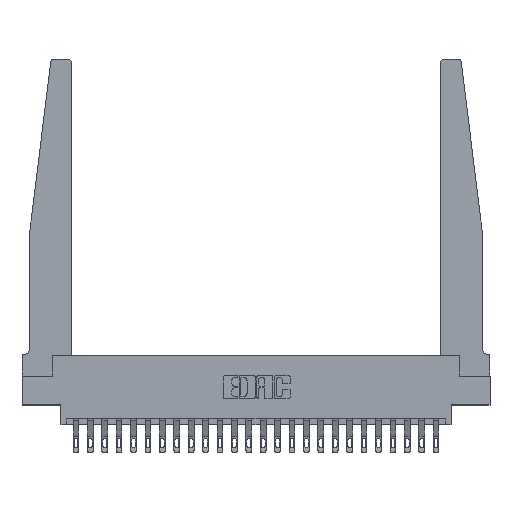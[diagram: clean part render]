
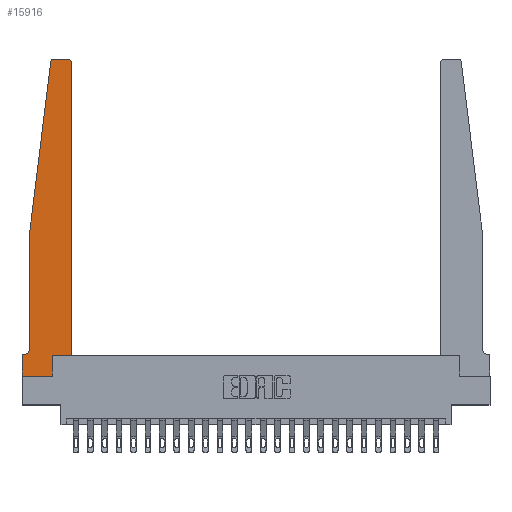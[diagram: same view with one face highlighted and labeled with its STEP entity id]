
A CAD part, top view. The second image highlights one B-rep face of the part: STEP entity #15916.
In plain terms, the highlighted planar face has unit normal (0, 0, 1).
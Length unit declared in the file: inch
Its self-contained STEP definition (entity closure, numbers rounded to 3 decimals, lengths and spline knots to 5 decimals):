
#28 = CARTESIAN_POINT ( 'NONE',  ( 0.015, 0.1875, 0.37 ) ) ;
#70 = LINE ( 'NONE', #19010, #5690 ) ;
#194 = DIRECTION ( 'NONE',  ( 0., 1., 0. ) ) ;
#240 = DIRECTION ( 'NONE',  ( 1., 0., 0. ) ) ;
#373 = ORIENTED_EDGE ( 'NONE', *, *, #10259, .T. ) ;
#909 = CIRCLE ( 'NONE', #4108, 0.05 ) ;
#1382 = CARTESIAN_POINT ( 'NONE',  ( 0.015, 0.2375, 0.37 ) ) ;
#1850 = LINE ( 'NONE', #20656, #7805 ) ;
#1872 = AXIS2_PLACEMENT_3D ( 'NONE', #8564, #6312, #14222 ) ;
#1913 = VECTOR ( 'NONE', #11447, 39.37008 ) ;
#2005 = VECTOR ( 'NONE', #15147, 39.37008 ) ;
#2633 = CIRCLE ( 'NONE', #9837, 0.03 ) ;
#2907 = FACE_OUTER_BOUND ( 'NONE', #6926, .T. ) ;
#2997 = CARTESIAN_POINT ( 'NONE',  ( 0.065, 0.2375, 0.37 ) ) ;
#3524 = CARTESIAN_POINT ( 'NONE',  ( 0., 0.1875, 0.37 ) ) ;
#4108 = AXIS2_PLACEMENT_3D ( 'NONE', #1382, #23730, #6535 ) ;
#4109 = EDGE_CURVE ( 'NONE', #15011, #24772, #13547, .T. ) ;
#5056 = VERTEX_POINT ( 'NONE', #17362 ) ;
#5690 = VECTOR ( 'NONE', #194, 39.37008 ) ;
#5766 = CARTESIAN_POINT ( 'NONE',  ( 0.27653, 2.72, 0.37 ) ) ;
#6125 = CARTESIAN_POINT ( 'NONE',  ( 0.395, 2.75, 0.37 ) ) ;
#6137 = VECTOR ( 'NONE', #12369, 39.37008 ) ;
#6312 = DIRECTION ( 'NONE',  ( 0., 0., 1. ) ) ;
#6467 = LINE ( 'NONE', #10232, #6137 ) ;
#6535 = DIRECTION ( 'NONE',  ( -1., 0., 0. ) ) ;
#6581 = ORIENTED_EDGE ( 'NONE', *, *, #11618, .T. ) ;
#6617 = CARTESIAN_POINT ( 'NONE',  ( 0.27653, 2.75, 0.37 ) ) ;
#6688 = EDGE_CURVE ( 'NONE', #13780, #5056, #14677, .T. ) ;
#6808 = CARTESIAN_POINT ( 'NONE',  ( 0.065, 1.25, 0.37 ) ) ;
#6926 = EDGE_LOOP ( 'NONE', ( #17609, #11077, #15080, #15619, #17497, #6581, #24684, #23770, #11872, #17098, #373, #19827 ) ) ;
#7206 = CARTESIAN_POINT ( 'NONE',  ( 0.425, 0.18, 0.37 ) ) ;
#7258 = EDGE_CURVE ( 'NONE', #12325, #13549, #1850, .T. ) ;
#7486 = CARTESIAN_POINT ( 'NONE',  ( 0.395, 2.72, 0.37 ) ) ;
#7602 = DIRECTION ( 'NONE',  ( -1., 0., 0. ) ) ;
#7733 = CARTESIAN_POINT ( 'NONE',  ( 0., 0., 0.37 ) ) ;
#7805 = VECTOR ( 'NONE', #11148, 39.37008 ) ;
#8400 = VERTEX_POINT ( 'NONE', #12075 ) ;
#8454 = CARTESIAN_POINT ( 'NONE',  ( 0.2605, 0.18, 0.37 ) ) ;
#8564 = CARTESIAN_POINT ( 'NONE',  ( 0., 0.1875, 0.37 ) ) ;
#8836 = VECTOR ( 'NONE', #7602, 39.37008 ) ;
#9041 = AXIS2_PLACEMENT_3D ( 'NONE', #5766, #12849, #10713 ) ;
#9180 = EDGE_CURVE ( 'NONE', #5056, #12325, #16848, .T. ) ;
#9837 = AXIS2_PLACEMENT_3D ( 'NONE', #7486, #13258, #19990 ) ;
#10232 = CARTESIAN_POINT ( 'NONE',  ( 0., 0., 0.37 ) ) ;
#10259 = EDGE_CURVE ( 'NONE', #24772, #8400, #70, .T. ) ;
#10713 = DIRECTION ( 'NONE',  ( 1., 0., 0. ) ) ;
#10812 = CARTESIAN_POINT ( 'NONE',  ( 0., 0., 0.37 ) ) ;
#10956 = CARTESIAN_POINT ( 'NONE',  ( 0.065, 1.25, 0.37 ) ) ;
#11077 = ORIENTED_EDGE ( 'NONE', *, *, #6688, .T. ) ;
#11148 = DIRECTION ( 'NONE',  ( 0., -1., 0. ) ) ;
#11172 = VERTEX_POINT ( 'NONE', #3524 ) ;
#11447 = DIRECTION ( 'NONE',  ( -0.122, -0.992, 0. ) ) ;
#11483 = LINE ( 'NONE', #20563, #8836 ) ;
#11560 = VECTOR ( 'NONE', #17736, 39.37008 ) ;
#11618 = EDGE_CURVE ( 'NONE', #12472, #11172, #21003, .T. ) ;
#11648 = CARTESIAN_POINT ( 'NONE',  ( 0.425, 0.18, 0.37 ) ) ;
#11737 = DIRECTION ( 'NONE',  ( -1., 0., 0. ) ) ;
#11742 = EDGE_CURVE ( 'NONE', #8400, #24030, #2633, .T. ) ;
#11872 = ORIENTED_EDGE ( 'NONE', *, *, #20787, .T. ) ;
#12075 = CARTESIAN_POINT ( 'NONE',  ( 0.425, 2.72, 0.37 ) ) ;
#12325 = VERTEX_POINT ( 'NONE', #6808 ) ;
#12369 = DIRECTION ( 'NONE',  ( 0., -1., 0. ) ) ;
#12472 = VERTEX_POINT ( 'NONE', #28 ) ;
#12849 = DIRECTION ( 'NONE',  ( 0., 0., 1. ) ) ;
#13258 = DIRECTION ( 'NONE',  ( 0., 0., 1. ) ) ;
#13417 = CARTESIAN_POINT ( 'NONE',  ( 0.2605, 0.18, 0.37 ) ) ;
#13547 = LINE ( 'NONE', #11648, #14205 ) ;
#13549 = VERTEX_POINT ( 'NONE', #2997 ) ;
#13772 = VERTEX_POINT ( 'NONE', #21028 ) ;
#13780 = VERTEX_POINT ( 'NONE', #6617 ) ;
#14205 = VECTOR ( 'NONE', #240, 39.37008 ) ;
#14222 = DIRECTION ( 'NONE',  ( 1., 0., 0. ) ) ;
#14225 = VERTEX_POINT ( 'NONE', #10812 ) ;
#14354 = PLANE ( 'NONE',  #1872 ) ;
#14677 = CIRCLE ( 'NONE', #9041, 0.03 ) ;
#15011 = VERTEX_POINT ( 'NONE', #13417 ) ;
#15080 = ORIENTED_EDGE ( 'NONE', *, *, #9180, .T. ) ;
#15147 = DIRECTION ( 'NONE',  ( 1., 0., 0. ) ) ;
#15619 = ORIENTED_EDGE ( 'NONE', *, *, #7258, .T. ) ;
#15916 = ADVANCED_FACE ( 'NONE', ( #2907 ), #14354, .T. ) ;
#16747 = EDGE_CURVE ( 'NONE', #11172, #14225, #6467, .T. ) ;
#16848 = LINE ( 'NONE', #10956, #1913 ) ;
#17098 = ORIENTED_EDGE ( 'NONE', *, *, #4109, .T. ) ;
#17362 = CARTESIAN_POINT ( 'NONE',  ( 0.24675, 2.72367, 0.37 ) ) ;
#17497 = ORIENTED_EDGE ( 'NONE', *, *, #19479, .T. ) ;
#17609 = ORIENTED_EDGE ( 'NONE', *, *, #23181, .T. ) ;
#17736 = DIRECTION ( 'NONE',  ( 0., 1., 0. ) ) ;
#18263 = VECTOR ( 'NONE', #11737, 39.37008 ) ;
#19010 = CARTESIAN_POINT ( 'NONE',  ( 0.425, 0.18, 0.37 ) ) ;
#19479 = EDGE_CURVE ( 'NONE', #13549, #12472, #909, .T. ) ;
#19827 = ORIENTED_EDGE ( 'NONE', *, *, #11742, .T. ) ;
#19990 = DIRECTION ( 'NONE',  ( 1., 0., 0. ) ) ;
#20218 = LINE ( 'NONE', #8454, #11560 ) ;
#20563 = CARTESIAN_POINT ( 'NONE',  ( 0.25, 2.75, 0.37 ) ) ;
#20656 = CARTESIAN_POINT ( 'NONE',  ( 0.065, 1.25, 0.37 ) ) ;
#20787 = EDGE_CURVE ( 'NONE', #13772, #15011, #20218, .T. ) ;
#20865 = LINE ( 'NONE', #7733, #2005 ) ;
#21003 = LINE ( 'NONE', #22895, #18263 ) ;
#21028 = CARTESIAN_POINT ( 'NONE',  ( 0.2605, 0., 0.37 ) ) ;
#22895 = CARTESIAN_POINT ( 'NONE',  ( 0.065, 0.1875, 0.37 ) ) ;
#23181 = EDGE_CURVE ( 'NONE', #24030, #13780, #11483, .T. ) ;
#23730 = DIRECTION ( 'NONE',  ( 0., 0., -1. ) ) ;
#23770 = ORIENTED_EDGE ( 'NONE', *, *, #24510, .T. ) ;
#24030 = VERTEX_POINT ( 'NONE', #6125 ) ;
#24510 = EDGE_CURVE ( 'NONE', #14225, #13772, #20865, .T. ) ;
#24684 = ORIENTED_EDGE ( 'NONE', *, *, #16747, .T. ) ;
#24772 = VERTEX_POINT ( 'NONE', #7206 ) ;
